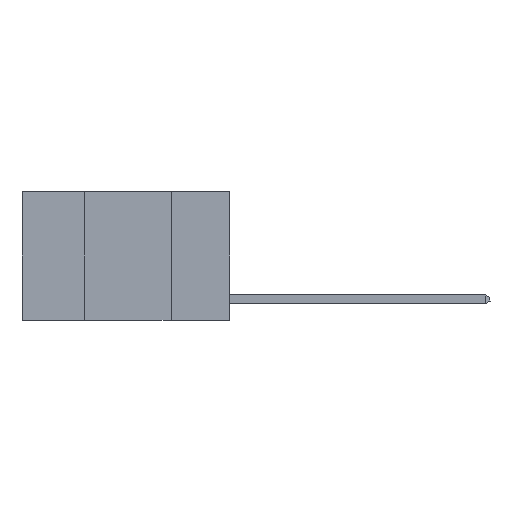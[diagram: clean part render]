
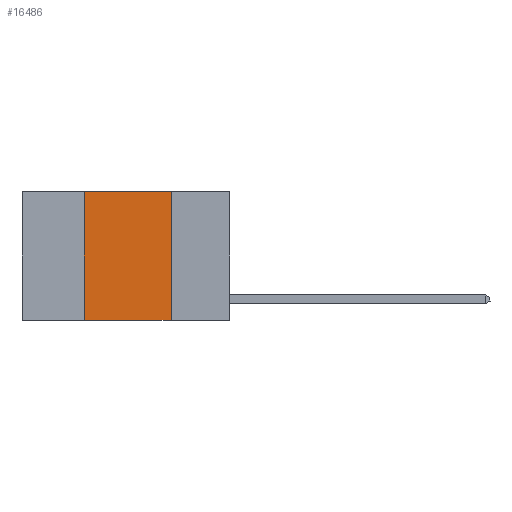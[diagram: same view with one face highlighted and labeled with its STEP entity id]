
A CAD part, left-side view. The second image highlights one B-rep face of the part: STEP entity #16486.
In plain terms, the highlighted planar face has unit normal (-1, 0, 0).
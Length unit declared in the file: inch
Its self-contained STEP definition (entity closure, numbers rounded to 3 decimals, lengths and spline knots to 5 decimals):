
#83 = VERTEX_POINT ( 'NONE', #9395 ) ;
#1123 = VERTEX_POINT ( 'NONE', #13098 ) ;
#2144 = DIRECTION ( 'NONE',  ( 0., -1., 0. ) ) ;
#2665 = PLANE ( 'NONE',  #16471 ) ;
#2782 = VECTOR ( 'NONE', #18549, 39.37008 ) ;
#3601 = EDGE_CURVE ( 'NONE', #4030, #16447, #6689, .T. ) ;
#4030 = VERTEX_POINT ( 'NONE', #16652 ) ;
#4158 = DIRECTION ( 'NONE',  ( 1., 0., 0. ) ) ;
#4684 = ORIENTED_EDGE ( 'NONE', *, *, #3601, .T. ) ;
#4938 = ORIENTED_EDGE ( 'NONE', *, *, #14853, .F. ) ;
#5301 = VECTOR ( 'NONE', #6472, 39.37008 ) ;
#5486 = CARTESIAN_POINT ( 'NONE',  ( 0., 0.17, -0.37 ) ) ;
#6380 = CARTESIAN_POINT ( 'NONE',  ( 0., 0.42, 0. ) ) ;
#6472 = DIRECTION ( 'NONE',  ( 0., 0., -1. ) ) ;
#6689 = LINE ( 'NONE', #12680, #2782 ) ;
#7035 = CARTESIAN_POINT ( 'NONE',  ( 0., 0.6, 0. ) ) ;
#7857 = DIRECTION ( 'NONE',  ( 0., 0., 1. ) ) ;
#8206 = EDGE_LOOP ( 'NONE', ( #16035, #13642, #4938, #4684 ) ) ;
#8581 = VECTOR ( 'NONE', #7857, 39.37008 ) ;
#8740 = LINE ( 'NONE', #12362, #12134 ) ;
#9395 = CARTESIAN_POINT ( 'NONE',  ( 0., 0.42, 0. ) ) ;
#9614 = LINE ( 'NONE', #16665, #5301 ) ;
#10657 = EDGE_CURVE ( 'NONE', #83, #1123, #8740, .T. ) ;
#12134 = VECTOR ( 'NONE', #2144, 39.37008 ) ;
#12362 = CARTESIAN_POINT ( 'NONE',  ( 0., 0.6, 0. ) ) ;
#12680 = CARTESIAN_POINT ( 'NONE',  ( 0., 0.6, -0.37 ) ) ;
#12806 = FACE_OUTER_BOUND ( 'NONE', #8206, .T. ) ;
#12888 = LINE ( 'NONE', #6380, #8581 ) ;
#13098 = CARTESIAN_POINT ( 'NONE',  ( 0., 0.17, 0. ) ) ;
#13642 = ORIENTED_EDGE ( 'NONE', *, *, #10657, .F. ) ;
#14332 = DIRECTION ( 'NONE',  ( 0., 0., -1. ) ) ;
#14853 = EDGE_CURVE ( 'NONE', #4030, #83, #12888, .T. ) ;
#16035 = ORIENTED_EDGE ( 'NONE', *, *, #16229, .F. ) ;
#16229 = EDGE_CURVE ( 'NONE', #1123, #16447, #9614, .T. ) ;
#16447 = VERTEX_POINT ( 'NONE', #5486 ) ;
#16471 = AXIS2_PLACEMENT_3D ( 'NONE', #7035, #4158, #14332 ) ;
#16486 = ADVANCED_FACE ( 'NONE', ( #12806 ), #2665, .F. ) ;
#16652 = CARTESIAN_POINT ( 'NONE',  ( 0., 0.42, -0.37 ) ) ;
#16665 = CARTESIAN_POINT ( 'NONE',  ( 0., 0.17, 0. ) ) ;
#18549 = DIRECTION ( 'NONE',  ( 0., -1., 0. ) ) ;
